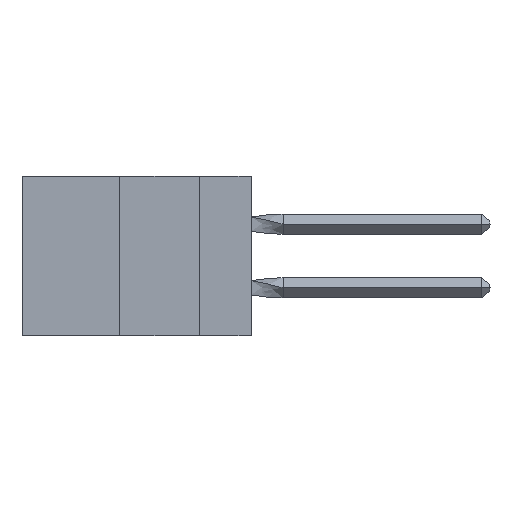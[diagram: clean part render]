
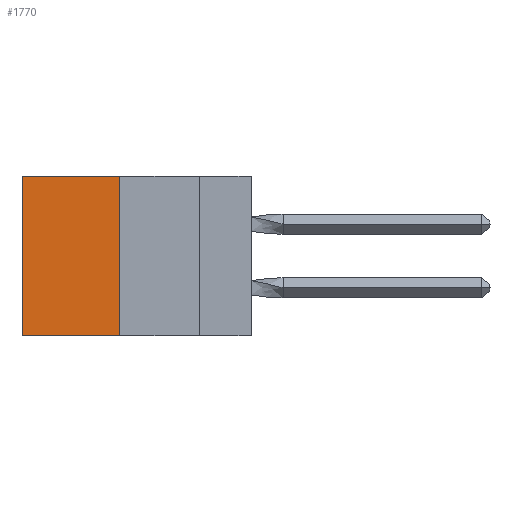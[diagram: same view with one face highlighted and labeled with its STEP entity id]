
A CAD part, left-side view. The second image highlights one B-rep face of the part: STEP entity #1770.
In plain terms, the highlighted planar face has unit normal (-1, 0, 0).
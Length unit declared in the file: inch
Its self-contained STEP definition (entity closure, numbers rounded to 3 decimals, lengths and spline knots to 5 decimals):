
#1415 = DIRECTION ( 'NONE',  ( 0., 0., -1. ) ) ;
#1445 = VECTOR ( 'NONE', #2412, 39.37008 ) ;
#1450 = AXIS2_PLACEMENT_3D ( 'NONE', #4488, #2991, #1415 ) ;
#1770 = ADVANCED_FACE ( 'NONE', ( #18168 ), #9153, .F. ) ;
#2193 = DIRECTION ( 'NONE',  ( 0., 0., -1. ) ) ;
#2412 = DIRECTION ( 'NONE',  ( 0., 1., 0. ) ) ;
#2991 = DIRECTION ( 'NONE',  ( 1., 0., 0. ) ) ;
#3129 = VECTOR ( 'NONE', #15921, 39.37008 ) ;
#3231 = VERTEX_POINT ( 'NONE', #16134 ) ;
#4092 = LINE ( 'NONE', #8375, #3129 ) ;
#4231 = VERTEX_POINT ( 'NONE', #15520 ) ;
#4488 = CARTESIAN_POINT ( 'NONE',  ( 0.305, 0.413, -0.5 ) ) ;
#4836 = LINE ( 'NONE', #12922, #13063 ) ;
#5357 = ORIENTED_EDGE ( 'NONE', *, *, #12139, .F. ) ;
#6321 = EDGE_CURVE ( 'NONE', #9887, #11174, #18962, .T. ) ;
#7176 = CARTESIAN_POINT ( 'NONE',  ( 0.305, 0.413, 0. ) ) ;
#8062 = CARTESIAN_POINT ( 'NONE',  ( 0.305, 0.72, 0. ) ) ;
#8375 = CARTESIAN_POINT ( 'NONE',  ( 0.305, 0.72, -0.5 ) ) ;
#9153 = PLANE ( 'NONE',  #1450 ) ;
#9887 = VERTEX_POINT ( 'NONE', #15446 ) ;
#11174 = VERTEX_POINT ( 'NONE', #8062 ) ;
#12139 = EDGE_CURVE ( 'NONE', #3231, #4231, #19134, .T. ) ;
#12922 = CARTESIAN_POINT ( 'NONE',  ( 0.305, 0.413, -0.5 ) ) ;
#13063 = VECTOR ( 'NONE', #2193, 39.37008 ) ;
#13319 = CARTESIAN_POINT ( 'NONE',  ( 0.305, 0.413, -0.5 ) ) ;
#15446 = CARTESIAN_POINT ( 'NONE',  ( 0.305, 0.413, 0. ) ) ;
#15520 = CARTESIAN_POINT ( 'NONE',  ( 0.305, 0.72, -0.5 ) ) ;
#15566 = ORIENTED_EDGE ( 'NONE', *, *, #19183, .F. ) ;
#15588 = VECTOR ( 'NONE', #18187, 39.37008 ) ;
#15921 = DIRECTION ( 'NONE',  ( 0., 0., -1. ) ) ;
#16134 = CARTESIAN_POINT ( 'NONE',  ( 0.305, 0.413, -0.5 ) ) ;
#17631 = EDGE_LOOP ( 'NONE', ( #18667, #5357, #15566, #18445 ) ) ;
#18168 = FACE_OUTER_BOUND ( 'NONE', #17631, .T. ) ;
#18187 = DIRECTION ( 'NONE',  ( 0., 1., 0. ) ) ;
#18445 = ORIENTED_EDGE ( 'NONE', *, *, #6321, .T. ) ;
#18667 = ORIENTED_EDGE ( 'NONE', *, *, #19268, .T. ) ;
#18962 = LINE ( 'NONE', #7176, #15588 ) ;
#19134 = LINE ( 'NONE', #13319, #1445 ) ;
#19183 = EDGE_CURVE ( 'NONE', #9887, #3231, #4836, .T. ) ;
#19268 = EDGE_CURVE ( 'NONE', #11174, #4231, #4092, .T. ) ;
